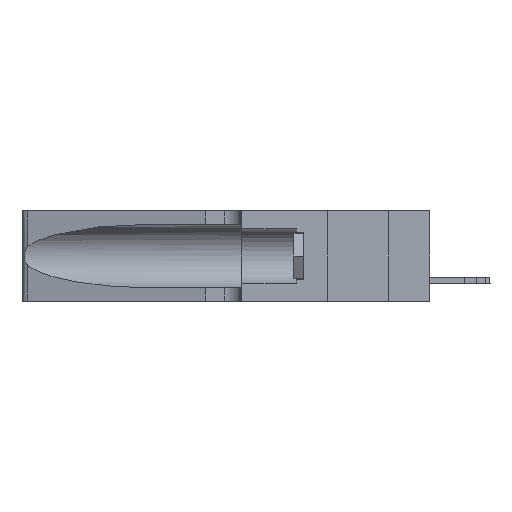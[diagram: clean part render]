
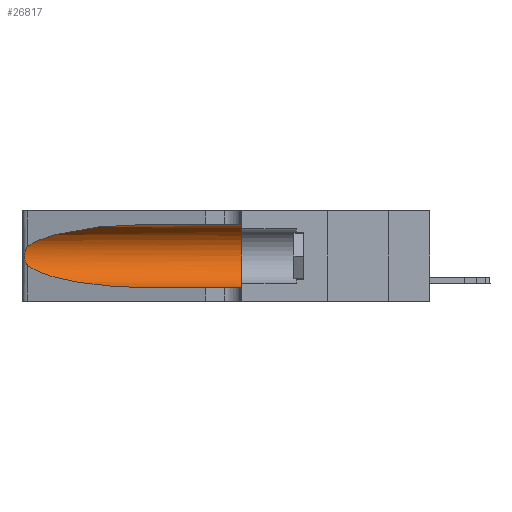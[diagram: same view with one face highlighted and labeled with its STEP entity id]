
A CAD part, left-side view. The second image highlights one B-rep face of the part: STEP entity #26817.
In plain terms, the highlighted cylindrical face has radius 3.308 mm (diameter 6.617 mm), a partial arc.
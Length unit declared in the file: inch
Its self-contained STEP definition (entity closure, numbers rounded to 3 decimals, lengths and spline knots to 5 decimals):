
#201 = CARTESIAN_POINT ( 'NONE',  ( 0.25487, 1.22718, 0.22369 ) ) ;
#934 = CARTESIAN_POINT ( 'NONE',  ( 0.1305, 0.72297, 0.31525 ) ) ;
#2202 = CARTESIAN_POINT ( 'NONE',  ( 0.25854, 1.2359, 0.20912 ) ) ;
#2382 = CARTESIAN_POINT ( 'NONE',  ( 0.1305, 0.72297, 0.05475 ) ) ;
#4712 = ORIENTED_EDGE ( 'NONE', *, *, #6092, .F. ) ;
#4924 = CARTESIAN_POINT ( 'NONE',  ( 0.26018, 1.23835, 0.19895 ) ) ;
#5047 = CARTESIAN_POINT ( 'NONE',  ( 0.25555, 1.22994, 0.2215 ) ) ;
#5773 =( BOUNDED_CURVE ( )  B_SPLINE_CURVE ( 3, ( #35310, #15670, #32516, #16152 ),
 .UNSPECIFIED., .F., .F. ) 
 B_SPLINE_CURVE_WITH_KNOTS ( ( 4, 4 ),
 ( 3.44316, 4.71239 ),
 .UNSPECIFIED. ) 
 CURVE ( )  GEOMETRIC_REPRESENTATION_ITEM ( )  RATIONAL_B_SPLINE_CURVE ( ( 1., 0.87, 0.87, 1. ) ) 
 REPRESENTATION_ITEM ( '' )  );
#5810 = EDGE_CURVE ( 'NONE', #31989, #17254, #20599, .T. ) ;
#6092 = EDGE_CURVE ( 'NONE', #31365, #13959, #6217, .T. ) ;
#6217 = CIRCLE ( 'NONE', #15316, 0.13025 ) ;
#6476 = CARTESIAN_POINT ( 'NONE',  ( 0.1305, 1.61858, 0.185 ) ) ;
#7290 = CARTESIAN_POINT ( 'NONE',  ( 0.25487, 1.22718, 0.14631 ) ) ;
#7827 = CARTESIAN_POINT ( 'NONE',  ( 0.25639, 1.23186, 0.15144 ) ) ;
#8351 = CARTESIAN_POINT ( 'NONE',  ( 0.2373, 1.15595, 0.28018 ) ) ;
#8578 = DIRECTION ( 'NONE',  ( 0., 1., 0. ) ) ;
#8653 = VECTOR ( 'NONE', #30092, 39.37008 ) ;
#9413 = ORIENTED_EDGE ( 'NONE', *, *, #15565, .T. ) ;
#9675 = ORIENTED_EDGE ( 'NONE', *, *, #5810, .T. ) ;
#10061 = VERTEX_POINT ( 'NONE', #2382 ) ;
#10735 = CARTESIAN_POINT ( 'NONE',  ( 0.25787, 1.23484, 0.2124 ) ) ;
#11352 = CARTESIAN_POINT ( 'NONE',  ( 0.1305, 0.72297, 0.31525 ) ) ;
#12406 = EDGE_CURVE ( 'NONE', #23088, #10061, #5773, .T. ) ;
#13080 = B_SPLINE_CURVE_WITH_KNOTS ( 'NONE', 3,
 ( #15805, #5047, #16044, #10735, #2202, #4924, #24238, #24361, #18585, #30029, #27007, #7827, #35442, #16299 ),
 .UNSPECIFIED., .F., .F.,
 ( 4, 2, 2, 2, 2, 2, 4 ),
 ( 0., 0.00027, 0.00053, 0.00107, 0.0016, 0.00187, 0.00214 ),
 .UNSPECIFIED. ) ;
#13959 = VERTEX_POINT ( 'NONE', #20024 ) ;
#15210 = CYLINDRICAL_SURFACE ( 'NONE', #29554, 0.13025 ) ;
#15316 = AXIS2_PLACEMENT_3D ( 'NONE', #25478, #8578, #30650 ) ;
#15565 = EDGE_CURVE ( 'NONE', #17254, #23088, #13080, .T. ) ;
#15670 = CARTESIAN_POINT ( 'NONE',  ( 0.2373, 1.15595, 0.08982 ) ) ;
#15805 = CARTESIAN_POINT ( 'NONE',  ( 0.25487, 1.22718, 0.22369 ) ) ;
#16044 = CARTESIAN_POINT ( 'NONE',  ( 0.25639, 1.23184, 0.21858 ) ) ;
#16152 = CARTESIAN_POINT ( 'NONE',  ( 0.1305, 0.72297, 0.05475 ) ) ;
#16299 = CARTESIAN_POINT ( 'NONE',  ( 0.25487, 1.22718, 0.14631 ) ) ;
#16821 = CARTESIAN_POINT ( 'NONE',  ( 0.18966, 0.96281, 0.31525 ) ) ;
#17254 = VERTEX_POINT ( 'NONE', #23447 ) ;
#18585 = CARTESIAN_POINT ( 'NONE',  ( 0.26017, 1.23833, 0.17102 ) ) ;
#18664 = FACE_OUTER_BOUND ( 'NONE', #24101, .T. ) ;
#20024 = CARTESIAN_POINT ( 'NONE',  ( 0.1305, 0.35, 0.05475 ) ) ;
#20599 =( BOUNDED_CURVE ( )  B_SPLINE_CURVE ( 3, ( #11352, #16821, #8351, #201 ),
 .UNSPECIFIED., .F., .F. ) 
 B_SPLINE_CURVE_WITH_KNOTS ( ( 4, 4 ),
 ( 1.5708, 2.84003 ),
 .UNSPECIFIED. ) 
 CURVE ( )  GEOMETRIC_REPRESENTATION_ITEM ( )  RATIONAL_B_SPLINE_CURVE ( ( 1., 0.87, 0.87, 1. ) ) 
 REPRESENTATION_ITEM ( '' )  );
#20795 = ORIENTED_EDGE ( 'NONE', *, *, #28554, .T. ) ;
#21959 = DIRECTION ( 'NONE',  ( 0., -1., 0. ) ) ;
#22821 = ORIENTED_EDGE ( 'NONE', *, *, #12406, .T. ) ;
#22887 = DIRECTION ( 'NONE',  ( 0., 0., -1. ) ) ;
#23088 = VERTEX_POINT ( 'NONE', #7290 ) ;
#23333 = LINE ( 'NONE', #32588, #8653 ) ;
#23447 = CARTESIAN_POINT ( 'NONE',  ( 0.25487, 1.22718, 0.22369 ) ) ;
#24101 = EDGE_LOOP ( 'NONE', ( #9675, #9413, #22821, #20795, #4712, #27325 ) ) ;
#24238 = CARTESIAN_POINT ( 'NONE',  ( 0.26075, 1.23896, 0.19203 ) ) ;
#24361 = CARTESIAN_POINT ( 'NONE',  ( 0.26075, 1.23896, 0.178 ) ) ;
#25478 = CARTESIAN_POINT ( 'NONE',  ( 0.1305, 0.35, 0.185 ) ) ;
#26736 = LINE ( 'NONE', #32905, #33142 ) ;
#26817 = ADVANCED_FACE ( 'NONE', ( #18664 ), #15210, .F. ) ;
#27007 = CARTESIAN_POINT ( 'NONE',  ( 0.25789, 1.23486, 0.15765 ) ) ;
#27325 = ORIENTED_EDGE ( 'NONE', *, *, #29202, .F. ) ;
#28554 = EDGE_CURVE ( 'NONE', #10061, #13959, #23333, .T. ) ;
#29202 = EDGE_CURVE ( 'NONE', #31989, #31365, #26736, .T. ) ;
#29554 = AXIS2_PLACEMENT_3D ( 'NONE', #6476, #33709, #22887 ) ;
#30029 = CARTESIAN_POINT ( 'NONE',  ( 0.25856, 1.23593, 0.16098 ) ) ;
#30092 = DIRECTION ( 'NONE',  ( 0., -1., 0. ) ) ;
#30650 = DIRECTION ( 'NONE',  ( 0., 0., 1. ) ) ;
#31365 = VERTEX_POINT ( 'NONE', #34173 ) ;
#31989 = VERTEX_POINT ( 'NONE', #934 ) ;
#32516 = CARTESIAN_POINT ( 'NONE',  ( 0.18966, 0.96281, 0.05475 ) ) ;
#32588 = CARTESIAN_POINT ( 'NONE',  ( 0.1305, 1.61858, 0.05475 ) ) ;
#32905 = CARTESIAN_POINT ( 'NONE',  ( 0.1305, 1.61858, 0.31525 ) ) ;
#33142 = VECTOR ( 'NONE', #21959, 39.37008 ) ;
#33709 = DIRECTION ( 'NONE',  ( 0., -1., 0. ) ) ;
#34173 = CARTESIAN_POINT ( 'NONE',  ( 0.1305, 0.35, 0.31525 ) ) ;
#35310 = CARTESIAN_POINT ( 'NONE',  ( 0.25487, 1.22718, 0.14631 ) ) ;
#35442 = CARTESIAN_POINT ( 'NONE',  ( 0.25555, 1.22993, 0.14849 ) ) ;
